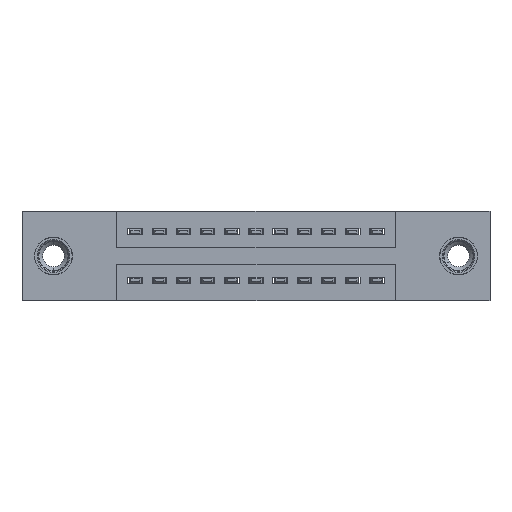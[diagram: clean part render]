
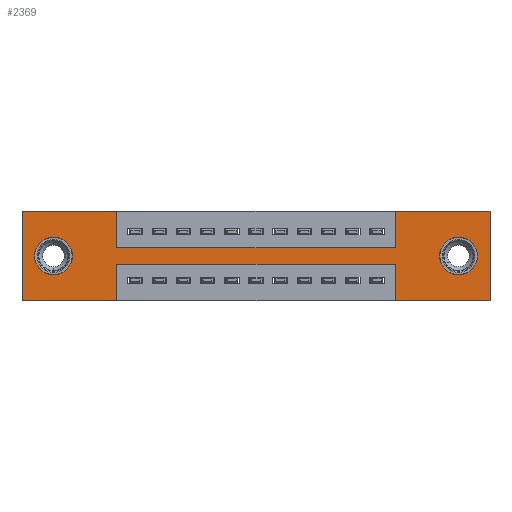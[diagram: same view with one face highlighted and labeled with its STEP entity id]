
A CAD part, front view. The second image highlights one B-rep face of the part: STEP entity #2369.
In plain terms, the highlighted planar face has unit normal (0, -1, 0).
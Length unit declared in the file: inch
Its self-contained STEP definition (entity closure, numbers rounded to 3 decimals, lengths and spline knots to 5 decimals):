
#186 = DIRECTION ( 'NONE',  ( 0., 0., -1. ) ) ;
#274 = AXIS2_PLACEMENT_3D ( 'NONE', #752, #9382, #13566 ) ;
#409 = AXIS2_PLACEMENT_3D ( 'NONE', #13079, #13127, #7720 ) ;
#525 = EDGE_CURVE ( 'NONE', #3010, #7239, #4489, .T. ) ;
#728 = DIRECTION ( 'NONE',  ( -1., 0., 0. ) ) ;
#752 = CARTESIAN_POINT ( 'NONE',  ( 1.805, 0., -0.185 ) ) ;
#777 = EDGE_CURVE ( 'NONE', #4770, #3636, #10982, .T. ) ;
#936 = CARTESIAN_POINT ( 'NONE',  ( 0.13, 0., -0.107 ) ) ;
#983 = ORIENTED_EDGE ( 'NONE', *, *, #777, .F. ) ;
#1175 = CIRCLE ( 'NONE', #8364, 0.078 ) ;
#1422 = AXIS2_PLACEMENT_3D ( 'NONE', #2895, #10357, #2766 ) ;
#1445 = ORIENTED_EDGE ( 'NONE', *, *, #12082, .F. ) ;
#1543 = CARTESIAN_POINT ( 'NONE',  ( 1.805, 0., -0.263 ) ) ;
#1553 = ORIENTED_EDGE ( 'NONE', *, *, #5233, .T. ) ;
#1580 = VERTEX_POINT ( 'NONE', #5528 ) ;
#1810 = CARTESIAN_POINT ( 'NONE',  ( 0., 0., -0.37 ) ) ;
#1899 = VERTEX_POINT ( 'NONE', #9079 ) ;
#2037 = CARTESIAN_POINT ( 'NONE',  ( 0.3925, 0., -0.22 ) ) ;
#2099 = CARTESIAN_POINT ( 'NONE',  ( 0.3925, 0., -0.15 ) ) ;
#2240 = EDGE_LOOP ( 'NONE', ( #1553, #6443 ) ) ;
#2369 = ADVANCED_FACE ( 'NONE', ( #3952, #8283, #7959 ), #9747, .T. ) ;
#2766 = DIRECTION ( 'NONE',  ( 0., 0., 1. ) ) ;
#2885 = EDGE_CURVE ( 'NONE', #7239, #1899, #4757, .T. ) ;
#2895 = CARTESIAN_POINT ( 'NONE',  ( 0.13, 0., -0.185 ) ) ;
#2950 = CARTESIAN_POINT ( 'NONE',  ( 1.5425, 0., -0.37 ) ) ;
#3010 = VERTEX_POINT ( 'NONE', #13057 ) ;
#3212 = VERTEX_POINT ( 'NONE', #3924 ) ;
#3296 = EDGE_CURVE ( 'NONE', #1580, #3212, #13711, .T. ) ;
#3523 = CARTESIAN_POINT ( 'NONE',  ( 1.5425, 0., -0.22 ) ) ;
#3606 = AXIS2_PLACEMENT_3D ( 'NONE', #5562, #9840, #4482 ) ;
#3636 = VERTEX_POINT ( 'NONE', #3523 ) ;
#3800 = CIRCLE ( 'NONE', #3606, 0.078 ) ;
#3924 = CARTESIAN_POINT ( 'NONE',  ( 0., 0., -0.37 ) ) ;
#3952 = FACE_BOUND ( 'NONE', #13311, .T. ) ;
#4072 = VERTEX_POINT ( 'NONE', #5464 ) ;
#4149 = CARTESIAN_POINT ( 'NONE',  ( 0.3925, 0., -0.37 ) ) ;
#4371 = ORIENTED_EDGE ( 'NONE', *, *, #6386, .F. ) ;
#4482 = DIRECTION ( 'NONE',  ( 0., 0., 1. ) ) ;
#4489 = LINE ( 'NONE', #6067, #9822 ) ;
#4611 = VERTEX_POINT ( 'NONE', #7151 ) ;
#4702 = CARTESIAN_POINT ( 'NONE',  ( 1.805, 0., -0.107 ) ) ;
#4711 = LINE ( 'NONE', #6869, #10691 ) ;
#4757 = LINE ( 'NONE', #8665, #12884 ) ;
#4770 = VERTEX_POINT ( 'NONE', #2950 ) ;
#4823 = ORIENTED_EDGE ( 'NONE', *, *, #8172, .F. ) ;
#4898 = ORIENTED_EDGE ( 'NONE', *, *, #13252, .F. ) ;
#4911 = VERTEX_POINT ( 'NONE', #9613 ) ;
#4925 = VERTEX_POINT ( 'NONE', #2099 ) ;
#4993 = VECTOR ( 'NONE', #11295, 39.37008 ) ;
#5233 = EDGE_CURVE ( 'NONE', #9337, #9164, #12410, .T. ) ;
#5238 = VECTOR ( 'NONE', #728, 39.37008 ) ;
#5352 = VECTOR ( 'NONE', #8006, 39.37008 ) ;
#5464 = CARTESIAN_POINT ( 'NONE',  ( 0.3925, 0., 0. ) ) ;
#5528 = CARTESIAN_POINT ( 'NONE',  ( 0.3925, 0., -0.37 ) ) ;
#5562 = CARTESIAN_POINT ( 'NONE',  ( 0.13, 0., -0.185 ) ) ;
#5762 = CARTESIAN_POINT ( 'NONE',  ( 0., 0., 0. ) ) ;
#5817 = DIRECTION ( 'NONE',  ( 1., 0., 0. ) ) ;
#5837 = LINE ( 'NONE', #10229, #12485 ) ;
#6067 = CARTESIAN_POINT ( 'NONE',  ( 1.5425, 0., 0. ) ) ;
#6245 = DIRECTION ( 'NONE',  ( 0., 0., -1. ) ) ;
#6377 = LINE ( 'NONE', #4149, #12373 ) ;
#6386 = EDGE_CURVE ( 'NONE', #12279, #1580, #6377, .T. ) ;
#6443 = ORIENTED_EDGE ( 'NONE', *, *, #9687, .T. ) ;
#6520 = ORIENTED_EDGE ( 'NONE', *, *, #3296, .F. ) ;
#6615 = CARTESIAN_POINT ( 'NONE',  ( 0.3925, 0., 0. ) ) ;
#6869 = CARTESIAN_POINT ( 'NONE',  ( 0., 0., 0. ) ) ;
#6959 = ORIENTED_EDGE ( 'NONE', *, *, #9269, .T. ) ;
#7026 = LINE ( 'NONE', #6615, #8671 ) ;
#7151 = CARTESIAN_POINT ( 'NONE',  ( 0., 0., 0. ) ) ;
#7239 = VERTEX_POINT ( 'NONE', #13823 ) ;
#7406 = CARTESIAN_POINT ( 'NONE',  ( 0.3925, 0., -0.15 ) ) ;
#7468 = VERTEX_POINT ( 'NONE', #1543 ) ;
#7720 = DIRECTION ( 'NONE',  ( 0., 0., -1. ) ) ;
#7959 = FACE_OUTER_BOUND ( 'NONE', #8509, .T. ) ;
#8006 = DIRECTION ( 'NONE',  ( 0., 0., 1. ) ) ;
#8061 = DIRECTION ( 'NONE',  ( 0., 1., 0. ) ) ;
#8136 = EDGE_CURVE ( 'NONE', #4911, #4770, #9827, .T. ) ;
#8172 = EDGE_CURVE ( 'NONE', #1899, #4911, #5837, .T. ) ;
#8259 = EDGE_CURVE ( 'NONE', #4925, #3010, #13643, .T. ) ;
#8283 = FACE_BOUND ( 'NONE', #2240, .T. ) ;
#8355 = ORIENTED_EDGE ( 'NONE', *, *, #8259, .F. ) ;
#8364 = AXIS2_PLACEMENT_3D ( 'NONE', #9086, #8061, #11152 ) ;
#8431 = ORIENTED_EDGE ( 'NONE', *, *, #525, .F. ) ;
#8509 = EDGE_LOOP ( 'NONE', ( #4371, #11664, #983, #10847, #4823, #8550, #8431, #8355, #4898, #1445, #11620, #6520 ) ) ;
#8550 = ORIENTED_EDGE ( 'NONE', *, *, #2885, .F. ) ;
#8665 = CARTESIAN_POINT ( 'NONE',  ( 0., 0., 0. ) ) ;
#8671 = VECTOR ( 'NONE', #186, 39.37008 ) ;
#9079 = CARTESIAN_POINT ( 'NONE',  ( 1.935, 0., 0. ) ) ;
#9086 = CARTESIAN_POINT ( 'NONE',  ( 1.805, 0., -0.185 ) ) ;
#9145 = CIRCLE ( 'NONE', #274, 0.078 ) ;
#9164 = VERTEX_POINT ( 'NONE', #13476 ) ;
#9169 = CARTESIAN_POINT ( 'NONE',  ( 0., 0., -0.37 ) ) ;
#9269 = EDGE_CURVE ( 'NONE', #11410, #7468, #9145, .T. ) ;
#9337 = VERTEX_POINT ( 'NONE', #936 ) ;
#9382 = DIRECTION ( 'NONE',  ( 0., 1., 0. ) ) ;
#9494 = LINE ( 'NONE', #2037, #12806 ) ;
#9613 = CARTESIAN_POINT ( 'NONE',  ( 1.935, 0., -0.37 ) ) ;
#9687 = EDGE_CURVE ( 'NONE', #9164, #9337, #3800, .T. ) ;
#9747 = PLANE ( 'NONE',  #409 ) ;
#9822 = VECTOR ( 'NONE', #12396, 39.37008 ) ;
#9827 = LINE ( 'NONE', #9169, #12167 ) ;
#9840 = DIRECTION ( 'NONE',  ( 0., 1., 0. ) ) ;
#10167 = VECTOR ( 'NONE', #11601, 39.37008 ) ;
#10229 = CARTESIAN_POINT ( 'NONE',  ( 1.935, 0., 0. ) ) ;
#10357 = DIRECTION ( 'NONE',  ( 0., 1., 0. ) ) ;
#10598 = CARTESIAN_POINT ( 'NONE',  ( 0.3925, 0., -0.22 ) ) ;
#10691 = VECTOR ( 'NONE', #5817, 39.37008 ) ;
#10792 = DIRECTION ( 'NONE',  ( 1., 0., 0. ) ) ;
#10847 = ORIENTED_EDGE ( 'NONE', *, *, #8136, .F. ) ;
#10982 = LINE ( 'NONE', #11195, #4993 ) ;
#11152 = DIRECTION ( 'NONE',  ( 0., 0., -1. ) ) ;
#11195 = CARTESIAN_POINT ( 'NONE',  ( 1.5425, 0., -0.37 ) ) ;
#11205 = ORIENTED_EDGE ( 'NONE', *, *, #12095, .T. ) ;
#11295 = DIRECTION ( 'NONE',  ( 0., 0., 1. ) ) ;
#11410 = VERTEX_POINT ( 'NONE', #4702 ) ;
#11601 = DIRECTION ( 'NONE',  ( 1., 0., 0. ) ) ;
#11620 = ORIENTED_EDGE ( 'NONE', *, *, #12534, .F. ) ;
#11664 = ORIENTED_EDGE ( 'NONE', *, *, #12870, .F. ) ;
#12016 = LINE ( 'NONE', #5762, #5352 ) ;
#12082 = EDGE_CURVE ( 'NONE', #4611, #4072, #4711, .T. ) ;
#12095 = EDGE_CURVE ( 'NONE', #7468, #11410, #1175, .T. ) ;
#12167 = VECTOR ( 'NONE', #12450, 39.37008 ) ;
#12279 = VERTEX_POINT ( 'NONE', #10598 ) ;
#12373 = VECTOR ( 'NONE', #6245, 39.37008 ) ;
#12396 = DIRECTION ( 'NONE',  ( 0., 0., 1. ) ) ;
#12406 = DIRECTION ( 'NONE',  ( 0., 0., -1. ) ) ;
#12410 = CIRCLE ( 'NONE', #1422, 0.078 ) ;
#12450 = DIRECTION ( 'NONE',  ( -1., 0., 0. ) ) ;
#12485 = VECTOR ( 'NONE', #12406, 39.37008 ) ;
#12534 = EDGE_CURVE ( 'NONE', #3212, #4611, #12016, .T. ) ;
#12600 = DIRECTION ( 'NONE',  ( -1., 0., 0. ) ) ;
#12806 = VECTOR ( 'NONE', #12600, 39.37008 ) ;
#12870 = EDGE_CURVE ( 'NONE', #3636, #12279, #9494, .T. ) ;
#12884 = VECTOR ( 'NONE', #10792, 39.37008 ) ;
#13057 = CARTESIAN_POINT ( 'NONE',  ( 1.5425, 0., -0.15 ) ) ;
#13079 = CARTESIAN_POINT ( 'NONE',  ( 0., 0., -0.37 ) ) ;
#13127 = DIRECTION ( 'NONE',  ( 0., -1., 0. ) ) ;
#13252 = EDGE_CURVE ( 'NONE', #4072, #4925, #7026, .T. ) ;
#13311 = EDGE_LOOP ( 'NONE', ( #6959, #11205 ) ) ;
#13476 = CARTESIAN_POINT ( 'NONE',  ( 0.13, 0., -0.263 ) ) ;
#13566 = DIRECTION ( 'NONE',  ( 0., 0., -1. ) ) ;
#13643 = LINE ( 'NONE', #7406, #10167 ) ;
#13711 = LINE ( 'NONE', #1810, #5238 ) ;
#13823 = CARTESIAN_POINT ( 'NONE',  ( 1.5425, 0., 0. ) ) ;
